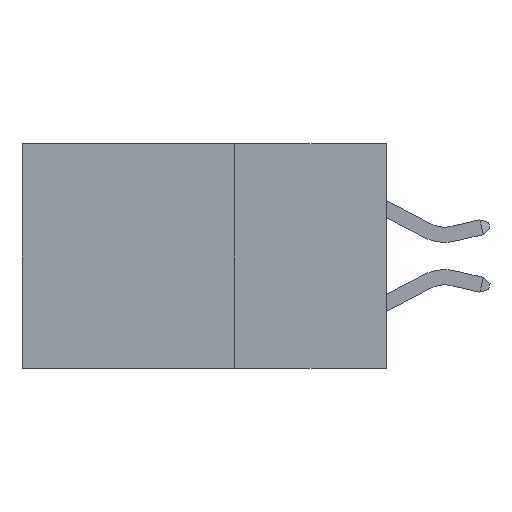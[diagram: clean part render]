
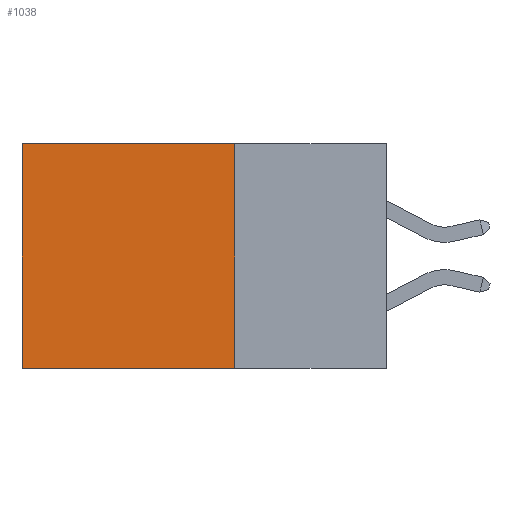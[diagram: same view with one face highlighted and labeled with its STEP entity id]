
A CAD part, left-side view. The second image highlights one B-rep face of the part: STEP entity #1038.
In plain terms, the highlighted planar face has unit normal (-1, 0, 0).
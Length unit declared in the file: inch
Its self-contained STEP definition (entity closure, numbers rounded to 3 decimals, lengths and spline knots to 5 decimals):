
#734 = PLANE ( 'NONE',  #6677 ) ;
#927 = CARTESIAN_POINT ( 'NONE',  ( 0.2615, 0.25, 0. ) ) ;
#1038 = ADVANCED_FACE ( 'NONE', ( #4536 ), #734, .F. ) ;
#1348 = EDGE_CURVE ( 'NONE', #7058, #9570, #3683, .T. ) ;
#1486 = LINE ( 'NONE', #6395, #7185 ) ;
#1572 = VECTOR ( 'NONE', #2221, 39.37008 ) ;
#1695 = ORIENTED_EDGE ( 'NONE', *, *, #5778, .T. ) ;
#1810 = CARTESIAN_POINT ( 'NONE',  ( 0.2615, 0.25, 0. ) ) ;
#1943 = LINE ( 'NONE', #6062, #9605 ) ;
#1987 = ORIENTED_EDGE ( 'NONE', *, *, #9024, .F. ) ;
#2001 = EDGE_CURVE ( 'NONE', #7058, #3710, #1943, .T. ) ;
#2042 = ORIENTED_EDGE ( 'NONE', *, *, #2001, .F. ) ;
#2221 = DIRECTION ( 'NONE',  ( 0., 1., 0. ) ) ;
#2454 = ORIENTED_EDGE ( 'NONE', *, *, #1348, .T. ) ;
#2552 = DIRECTION ( 'NONE',  ( 0., 0., -1. ) ) ;
#3136 = CARTESIAN_POINT ( 'NONE',  ( 0.2615, 0.25, -0.37 ) ) ;
#3683 = LINE ( 'NONE', #1810, #1572 ) ;
#3710 = VERTEX_POINT ( 'NONE', #5555 ) ;
#4536 = FACE_OUTER_BOUND ( 'NONE', #7437, .T. ) ;
#5159 = DIRECTION ( 'NONE',  ( 0., 0., -1. ) ) ;
#5555 = CARTESIAN_POINT ( 'NONE',  ( 0.2615, 0.25, -0.37 ) ) ;
#5593 = VECTOR ( 'NONE', #7001, 39.37008 ) ;
#5778 = EDGE_CURVE ( 'NONE', #9570, #6885, #1486, .T. ) ;
#6062 = CARTESIAN_POINT ( 'NONE',  ( 0.2615, 0.25, -0.37 ) ) ;
#6395 = CARTESIAN_POINT ( 'NONE',  ( 0.2615, 0.6, -0.37 ) ) ;
#6677 = AXIS2_PLACEMENT_3D ( 'NONE', #7344, #6977, #5159 ) ;
#6885 = VERTEX_POINT ( 'NONE', #8184 ) ;
#6977 = DIRECTION ( 'NONE',  ( 1., 0., 0. ) ) ;
#7001 = DIRECTION ( 'NONE',  ( 0., 1., 0. ) ) ;
#7058 = VERTEX_POINT ( 'NONE', #927 ) ;
#7185 = VECTOR ( 'NONE', #2552, 39.37008 ) ;
#7344 = CARTESIAN_POINT ( 'NONE',  ( 0.2615, 0.25, -0.37 ) ) ;
#7437 = EDGE_LOOP ( 'NONE', ( #1695, #1987, #2042, #2454 ) ) ;
#7633 = LINE ( 'NONE', #3136, #5593 ) ;
#8184 = CARTESIAN_POINT ( 'NONE',  ( 0.2615, 0.6, -0.37 ) ) ;
#8291 = DIRECTION ( 'NONE',  ( 0., 0., -1. ) ) ;
#9024 = EDGE_CURVE ( 'NONE', #3710, #6885, #7633, .T. ) ;
#9033 = CARTESIAN_POINT ( 'NONE',  ( 0.2615, 0.6, 0. ) ) ;
#9570 = VERTEX_POINT ( 'NONE', #9033 ) ;
#9605 = VECTOR ( 'NONE', #8291, 39.37008 ) ;
